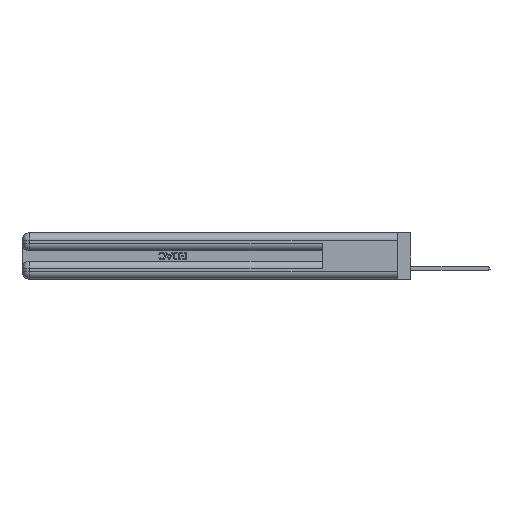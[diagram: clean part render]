
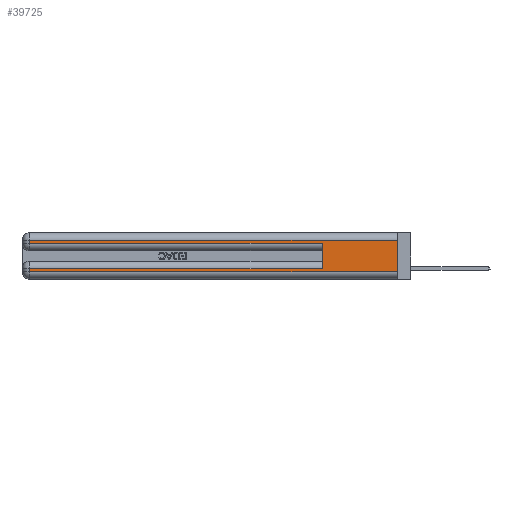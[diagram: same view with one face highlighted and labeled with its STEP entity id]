
A CAD part, left-side view. The second image highlights one B-rep face of the part: STEP entity #39725.
In plain terms, the highlighted planar face has unit normal (-1, 0, 0).
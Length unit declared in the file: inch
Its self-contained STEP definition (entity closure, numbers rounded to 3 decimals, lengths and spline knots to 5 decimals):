
#969 = VERTEX_POINT ( 'NONE', #4225 ) ;
#4225 = CARTESIAN_POINT ( 'NONE',  ( 0., 0., 0.06 ) ) ;
#5770 = LINE ( 'NONE', #35619, #6394 ) ;
#5786 = EDGE_CURVE ( 'NONE', #28403, #18916, #5770, .T. ) ;
#6330 = CARTESIAN_POINT ( 'NONE',  ( 0., 0., 0.06 ) ) ;
#6394 = VECTOR ( 'NONE', #31700, 39.37008 ) ;
#6731 = DIRECTION ( 'NONE',  ( 0., 0., -1. ) ) ;
#6750 = CARTESIAN_POINT ( 'NONE',  ( 0., 0., 0.085 ) ) ;
#7049 = AXIS2_PLACEMENT_3D ( 'NONE', #22676, #10899, #6731 ) ;
#7158 = LINE ( 'NONE', #16980, #47836 ) ;
#7705 = EDGE_CURVE ( 'NONE', #24064, #25206, #37817, .T. ) ;
#8724 = LINE ( 'NONE', #6750, #30432 ) ;
#10418 = EDGE_LOOP ( 'NONE', ( #11669, #26252, #38947, #35576, #19612, #25281, #40307, #11067 ) ) ;
#10899 = DIRECTION ( 'NONE',  ( 1., 0., 0. ) ) ;
#11067 = ORIENTED_EDGE ( 'NONE', *, *, #40284, .T. ) ;
#11669 = ORIENTED_EDGE ( 'NONE', *, *, #24952, .F. ) ;
#11727 = CARTESIAN_POINT ( 'NONE',  ( 0., 2.94, 0.06 ) ) ;
#14273 = DIRECTION ( 'NONE',  ( 0., -1., 0. ) ) ;
#15455 = VECTOR ( 'NONE', #23327, 39.37008 ) ;
#15774 = EDGE_CURVE ( 'NONE', #45174, #38151, #8724, .T. ) ;
#16679 = CARTESIAN_POINT ( 'NONE',  ( 0., 0.6, 0.285 ) ) ;
#16980 = CARTESIAN_POINT ( 'NONE',  ( 0., 2.94, 0.37 ) ) ;
#17632 = CARTESIAN_POINT ( 'NONE',  ( 0., 2.94, 0.285 ) ) ;
#18916 = VERTEX_POINT ( 'NONE', #16679 ) ;
#19612 = ORIENTED_EDGE ( 'NONE', *, *, #37516, .F. ) ;
#21391 = DIRECTION ( 'NONE',  ( 0., 0., -1. ) ) ;
#22260 = CARTESIAN_POINT ( 'NONE',  ( 0., 2.94, 0.31 ) ) ;
#22676 = CARTESIAN_POINT ( 'NONE',  ( 0., 0., 0.37 ) ) ;
#23327 = DIRECTION ( 'NONE',  ( 0., 0., 1. ) ) ;
#23391 = CARTESIAN_POINT ( 'NONE',  ( 0., 0., 0.37 ) ) ;
#24064 = VERTEX_POINT ( 'NONE', #28423 ) ;
#24430 = DIRECTION ( 'NONE',  ( 0., 0., -1. ) ) ;
#24952 = EDGE_CURVE ( 'NONE', #24064, #969, #49125, .T. ) ;
#25206 = VERTEX_POINT ( 'NONE', #22260 ) ;
#25281 = ORIENTED_EDGE ( 'NONE', *, *, #15774, .T. ) ;
#25285 = LINE ( 'NONE', #33766, #33291 ) ;
#25985 = CARTESIAN_POINT ( 'NONE',  ( 0., 0., 0.31 ) ) ;
#26014 = LINE ( 'NONE', #31062, #15455 ) ;
#26252 = ORIENTED_EDGE ( 'NONE', *, *, #7705, .T. ) ;
#28403 = VERTEX_POINT ( 'NONE', #17632 ) ;
#28423 = CARTESIAN_POINT ( 'NONE',  ( 0., 0., 0.31 ) ) ;
#29681 = CARTESIAN_POINT ( 'NONE',  ( 0., 2.94, 0.085 ) ) ;
#30432 = VECTOR ( 'NONE', #50056, 39.37008 ) ;
#30625 = DIRECTION ( 'NONE',  ( 0., 0., -1. ) ) ;
#31062 = CARTESIAN_POINT ( 'NONE',  ( 0., 0.6, 0.145 ) ) ;
#31700 = DIRECTION ( 'NONE',  ( 0., -1., 0. ) ) ;
#32333 = VECTOR ( 'NONE', #49747, 39.37008 ) ;
#33291 = VECTOR ( 'NONE', #21391, 39.37008 ) ;
#33766 = CARTESIAN_POINT ( 'NONE',  ( 0., 2.94, 0.37 ) ) ;
#34879 = VERTEX_POINT ( 'NONE', #11727 ) ;
#35576 = ORIENTED_EDGE ( 'NONE', *, *, #5786, .T. ) ;
#35619 = CARTESIAN_POINT ( 'NONE',  ( 0., 0., 0.285 ) ) ;
#37516 = EDGE_CURVE ( 'NONE', #45174, #18916, #26014, .T. ) ;
#37817 = LINE ( 'NONE', #25985, #32333 ) ;
#38066 = PLANE ( 'NONE',  #7049 ) ;
#38151 = VERTEX_POINT ( 'NONE', #29681 ) ;
#38162 = EDGE_CURVE ( 'NONE', #25206, #28403, #25285, .T. ) ;
#38591 = VECTOR ( 'NONE', #30625, 39.37008 ) ;
#38947 = ORIENTED_EDGE ( 'NONE', *, *, #38162, .T. ) ;
#39725 = ADVANCED_FACE ( 'NONE', ( #41066 ), #38066, .F. ) ;
#40284 = EDGE_CURVE ( 'NONE', #34879, #969, #44747, .T. ) ;
#40307 = ORIENTED_EDGE ( 'NONE', *, *, #45798, .T. ) ;
#40782 = CARTESIAN_POINT ( 'NONE',  ( 0., 0.6, 0.085 ) ) ;
#41066 = FACE_OUTER_BOUND ( 'NONE', #10418, .T. ) ;
#44747 = LINE ( 'NONE', #6330, #49064 ) ;
#45174 = VERTEX_POINT ( 'NONE', #40782 ) ;
#45798 = EDGE_CURVE ( 'NONE', #38151, #34879, #7158, .T. ) ;
#47836 = VECTOR ( 'NONE', #24430, 39.37008 ) ;
#49064 = VECTOR ( 'NONE', #14273, 39.37008 ) ;
#49125 = LINE ( 'NONE', #23391, #38591 ) ;
#49747 = DIRECTION ( 'NONE',  ( 0., 1., 0. ) ) ;
#50056 = DIRECTION ( 'NONE',  ( 0., 1., 0. ) ) ;
